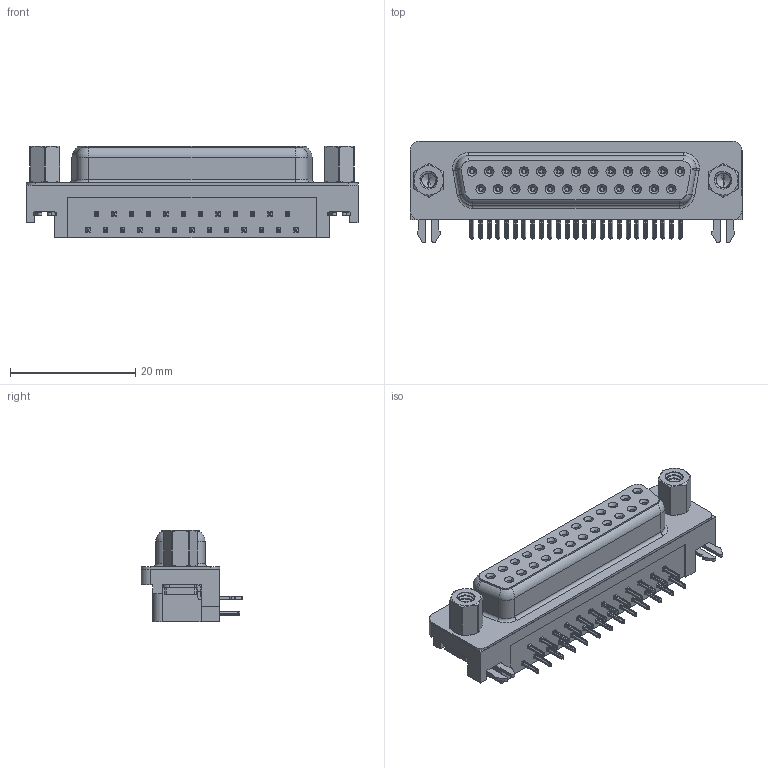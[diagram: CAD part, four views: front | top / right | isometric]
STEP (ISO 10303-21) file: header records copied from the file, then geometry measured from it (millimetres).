
FILE_DESCRIPTION (( 'STEP AP203' ), '1' );
FILE_NAME ('624-025-661-033.STEP', '2018-11-06T20:19:22', ( '' ), ( '' ), 'SwSTEP 2.0', 'SolidWorks 2016', '' );
FILE_SCHEMA (( 'CONFIG_CONTROL_DESIGN' ));
Length unit declared in the file: millimetre
Products named in the file (8): 624 Shell_25 Socket; 624 Socket Bottom; 624 Contact Top; 624 2 Prong Board Lock; 624 4-40 Threaded Rivet; 624 4-40 Hex Standoff 5; 624-025-661-033; 624 Housing_25 Socket
Assembly tree (33 placements, depth 2):
  624-025-661-033
    624 Housing_25 Socket
    624 Shell_25 Socket
    624 Socket Bottom  x12
    624 Contact Top  x13
    624 2 Prong Board Lock  x2
    624 4-40 Threaded Rivet  x2
    624 4-40 Hex Standoff 5  x2
Bounding box: 53.04 x 16.25 x 14.6 mm (x, y, z)
Volume: 6170.4 mm3; surface area: 8747.6 mm2
Topology: 33 solids, 33 shells, 3876 faces, 10238 edges, 6452 vertices
Faces by surface type: plane 1652, cylinder 982, bspline 870, cone 334, torus 38
Entity records: 35475 total; most frequent: CARTESIAN_POINT 12850, ORIENTED_EDGE 4534, DIRECTION 4072, EDGE_CURVE 2267, VERTEX_POINT 1452, LINE 1410, VECTOR 1410, AXIS2_PLACEMENT_3D 1331
